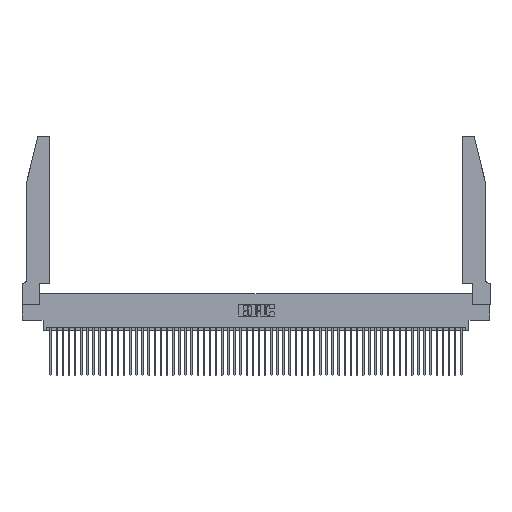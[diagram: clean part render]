
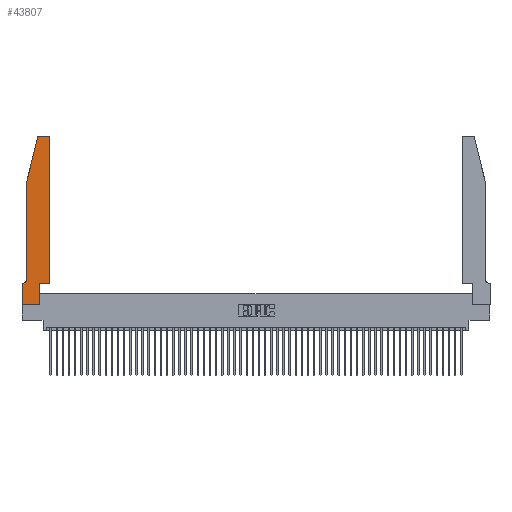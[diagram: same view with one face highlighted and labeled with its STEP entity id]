
A CAD part, top view. The second image highlights one B-rep face of the part: STEP entity #43807.
In plain terms, the highlighted planar face has unit normal (0, 0, 1).
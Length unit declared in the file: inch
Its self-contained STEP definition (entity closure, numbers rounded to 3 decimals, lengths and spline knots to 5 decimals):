
#37 = DIRECTION ( 'NONE',  ( 1., 0., 0. ) ) ;
#171 = DIRECTION ( 'NONE',  ( 0., 1., 0. ) ) ;
#561 = AXIS2_PLACEMENT_3D ( 'NONE', #11882, #41400, #16183 ) ;
#827 = LINE ( 'NONE', #24736, #44642 ) ;
#926 = DIRECTION ( 'NONE',  ( 0., -1., 0. ) ) ;
#1048 = CARTESIAN_POINT ( 'NONE',  ( 0.2865, 0.35, 0.37 ) ) ;
#1160 = EDGE_CURVE ( 'NONE', #22809, #3418, #10436, .T. ) ;
#1947 = CARTESIAN_POINT ( 'NONE',  ( 0.25487, 2.72718, 0.37 ) ) ;
#2196 = VERTEX_POINT ( 'NONE', #37077 ) ;
#3119 = CARTESIAN_POINT ( 'NONE',  ( 0.0755, 2., 0.37 ) ) ;
#3418 = VERTEX_POINT ( 'NONE', #15756 ) ;
#4562 = DIRECTION ( 'NONE',  ( 0., 0., -1. ) ) ;
#4904 = ORIENTED_EDGE ( 'NONE', *, *, #28595, .T. ) ;
#4944 = LINE ( 'NONE', #50915, #37457 ) ;
#4974 = LINE ( 'NONE', #3119, #48596 ) ;
#5139 = CARTESIAN_POINT ( 'NONE',  ( 0.0755, 2., 0.37 ) ) ;
#5278 = CARTESIAN_POINT ( 'NONE',  ( 0.4505, 0.35, 0.37 ) ) ;
#5665 = VERTEX_POINT ( 'NONE', #34879 ) ;
#6133 = CARTESIAN_POINT ( 'NONE',  ( 0.0755, 2., 0.37 ) ) ;
#7108 = ORIENTED_EDGE ( 'NONE', *, *, #15666, .T. ) ;
#7501 = EDGE_CURVE ( 'NONE', #12690, #5665, #33353, .T. ) ;
#8786 = LINE ( 'NONE', #43345, #31373 ) ;
#8894 = AXIS2_PLACEMENT_3D ( 'NONE', #30097, #4562, #34323 ) ;
#9061 = CARTESIAN_POINT ( 'NONE',  ( 0., 0., 0.37 ) ) ;
#9636 = DIRECTION ( 'NONE',  ( 1., 0., 0. ) ) ;
#10436 = LINE ( 'NONE', #5278, #23074 ) ;
#11882 = CARTESIAN_POINT ( 'NONE',  ( 0.4205, 2.72, 0.37 ) ) ;
#12121 = DIRECTION ( 'NONE',  ( 0., 1., 0. ) ) ;
#12563 = ORIENTED_EDGE ( 'NONE', *, *, #31056, .T. ) ;
#12690 = VERTEX_POINT ( 'NONE', #34751 ) ;
#13462 = CIRCLE ( 'NONE', #561, 0.03 ) ;
#14575 = LINE ( 'NONE', #32516, #48144 ) ;
#15666 = EDGE_CURVE ( 'NONE', #21738, #32679, #4974, .T. ) ;
#15756 = CARTESIAN_POINT ( 'NONE',  ( 0.4505, 0.35, 0.37 ) ) ;
#16076 = EDGE_CURVE ( 'NONE', #19524, #12690, #38752, .T. ) ;
#16183 = DIRECTION ( 'NONE',  ( 1., 0., 0. ) ) ;
#18018 = ORIENTED_EDGE ( 'NONE', *, *, #44231, .T. ) ;
#18198 = EDGE_CURVE ( 'NONE', #37261, #19524, #27473, .T. ) ;
#19320 = ORIENTED_EDGE ( 'NONE', *, *, #28918, .T. ) ;
#19524 = VERTEX_POINT ( 'NONE', #34223 ) ;
#20212 = DIRECTION ( 'NONE',  ( -0.239, -0.971, 0. ) ) ;
#20473 = VERTEX_POINT ( 'NONE', #48727 ) ;
#20822 = VECTOR ( 'NONE', #30240, 39.37008 ) ;
#21422 = ORIENTED_EDGE ( 'NONE', *, *, #1160, .T. ) ;
#21520 = PLANE ( 'NONE',  #50584 ) ;
#21738 = VERTEX_POINT ( 'NONE', #1947 ) ;
#22470 = DIRECTION ( 'NONE',  ( 1., 0., 0. ) ) ;
#22809 = VERTEX_POINT ( 'NONE', #1048 ) ;
#22940 = DIRECTION ( 'NONE',  ( -1., 0., 0. ) ) ;
#23074 = VECTOR ( 'NONE', #9636, 39.37008 ) ;
#24736 = CARTESIAN_POINT ( 'NONE',  ( 0.4505, 0.35, 0.37 ) ) ;
#25151 = EDGE_CURVE ( 'NONE', #48382, #21738, #25857, .T. ) ;
#25212 = EDGE_LOOP ( 'NONE', ( #18018, #54620, #7108, #19320, #27693, #41458, #54211, #44840, #44641, #21422, #4904, #12563 ) ) ;
#25533 = CARTESIAN_POINT ( 'NONE',  ( 0.284, 2.72, 0.37 ) ) ;
#25738 = DIRECTION ( 'NONE',  ( 0., 0., 1. ) ) ;
#25857 = CIRCLE ( 'NONE', #31486, 0.03 ) ;
#27473 = CIRCLE ( 'NONE', #8894, 0.07 ) ;
#27615 = VECTOR ( 'NONE', #22940, 39.37008 ) ;
#27693 = ORIENTED_EDGE ( 'NONE', *, *, #18198, .T. ) ;
#28595 = EDGE_CURVE ( 'NONE', #3418, #20473, #827, .T. ) ;
#28918 = EDGE_CURVE ( 'NONE', #32679, #37261, #43384, .T. ) ;
#29792 = DIRECTION ( 'NONE',  ( 1., 0., 0. ) ) ;
#30097 = CARTESIAN_POINT ( 'NONE',  ( 0.0055, 0.42, 0.37 ) ) ;
#30240 = DIRECTION ( 'NONE',  ( 0., -1., 0. ) ) ;
#30965 = VECTOR ( 'NONE', #926, 39.37008 ) ;
#31056 = EDGE_CURVE ( 'NONE', #20473, #54311, #13462, .T. ) ;
#31373 = VECTOR ( 'NONE', #22470, 39.37008 ) ;
#31486 = AXIS2_PLACEMENT_3D ( 'NONE', #25533, #54773, #29792 ) ;
#32516 = CARTESIAN_POINT ( 'NONE',  ( 0.2605, 2.75, 0.37 ) ) ;
#32679 = VERTEX_POINT ( 'NONE', #6133 ) ;
#33353 = LINE ( 'NONE', #9061, #20822 ) ;
#34223 = CARTESIAN_POINT ( 'NONE',  ( 0.0055, 0.35, 0.37 ) ) ;
#34323 = DIRECTION ( 'NONE',  ( -1., 0., 0. ) ) ;
#34675 = CARTESIAN_POINT ( 'NONE',  ( 0.4205, 2.75, 0.37 ) ) ;
#34751 = CARTESIAN_POINT ( 'NONE',  ( 0., 0.35, 0.37 ) ) ;
#34879 = CARTESIAN_POINT ( 'NONE',  ( 0., 0., 0.37 ) ) ;
#35779 = FACE_OUTER_BOUND ( 'NONE', #25212, .T. ) ;
#36908 = EDGE_CURVE ( 'NONE', #5665, #2196, #8786, .T. ) ;
#37077 = CARTESIAN_POINT ( 'NONE',  ( 0.2865, 0., 0.37 ) ) ;
#37261 = VERTEX_POINT ( 'NONE', #46198 ) ;
#37457 = VECTOR ( 'NONE', #171, 39.37008 ) ;
#38219 = CARTESIAN_POINT ( 'NONE',  ( 0., 0.35, 0.37 ) ) ;
#38752 = LINE ( 'NONE', #52211, #27615 ) ;
#41400 = DIRECTION ( 'NONE',  ( 0., 0., 1. ) ) ;
#41458 = ORIENTED_EDGE ( 'NONE', *, *, #16076, .T. ) ;
#43345 = CARTESIAN_POINT ( 'NONE',  ( 0., 0., 0.37 ) ) ;
#43384 = LINE ( 'NONE', #5139, #30965 ) ;
#43807 = ADVANCED_FACE ( 'NONE', ( #35779 ), #21520, .T. ) ;
#44231 = EDGE_CURVE ( 'NONE', #54311, #48382, #14575, .T. ) ;
#44641 = ORIENTED_EDGE ( 'NONE', *, *, #46265, .T. ) ;
#44642 = VECTOR ( 'NONE', #12121, 39.37008 ) ;
#44840 = ORIENTED_EDGE ( 'NONE', *, *, #36908, .T. ) ;
#46198 = CARTESIAN_POINT ( 'NONE',  ( 0.0755, 0.42, 0.37 ) ) ;
#46265 = EDGE_CURVE ( 'NONE', #2196, #22809, #4944, .T. ) ;
#48144 = VECTOR ( 'NONE', #49120, 39.37008 ) ;
#48382 = VERTEX_POINT ( 'NONE', #53017 ) ;
#48596 = VECTOR ( 'NONE', #20212, 39.37008 ) ;
#48727 = CARTESIAN_POINT ( 'NONE',  ( 0.4505, 2.72, 0.37 ) ) ;
#49120 = DIRECTION ( 'NONE',  ( -1., 0., 0. ) ) ;
#50584 = AXIS2_PLACEMENT_3D ( 'NONE', #38219, #25738, #37 ) ;
#50915 = CARTESIAN_POINT ( 'NONE',  ( 0.2865, 0.35, 0.37 ) ) ;
#52211 = CARTESIAN_POINT ( 'NONE',  ( 0.0755, 0.35, 0.37 ) ) ;
#53017 = CARTESIAN_POINT ( 'NONE',  ( 0.284, 2.75, 0.37 ) ) ;
#54211 = ORIENTED_EDGE ( 'NONE', *, *, #7501, .T. ) ;
#54311 = VERTEX_POINT ( 'NONE', #34675 ) ;
#54620 = ORIENTED_EDGE ( 'NONE', *, *, #25151, .T. ) ;
#54773 = DIRECTION ( 'NONE',  ( 0., 0., 1. ) ) ;
